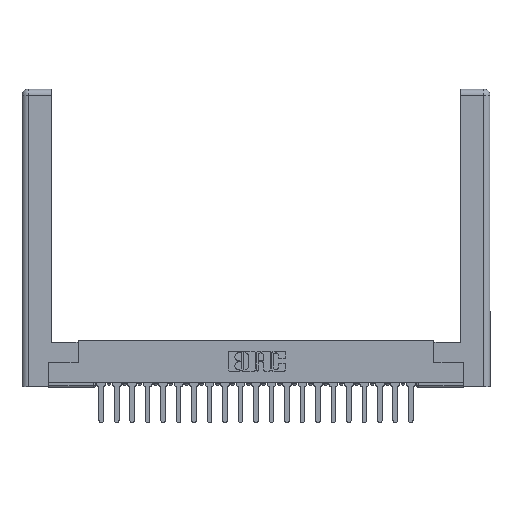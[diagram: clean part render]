
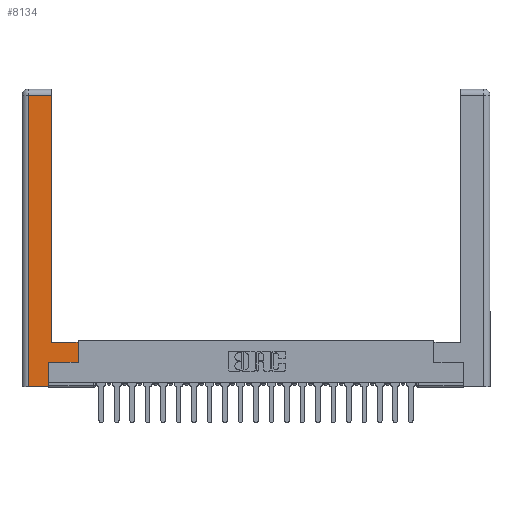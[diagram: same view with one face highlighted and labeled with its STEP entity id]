
A CAD part, top view. The second image highlights one B-rep face of the part: STEP entity #8134.
In plain terms, the highlighted planar face has unit normal (0, 0, 1).
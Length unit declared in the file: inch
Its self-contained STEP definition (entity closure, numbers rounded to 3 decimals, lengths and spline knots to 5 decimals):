
#376 = EDGE_CURVE ( 'NONE', #17551, #21999, #12902, .T. ) ;
#1391 = CARTESIAN_POINT ( 'NONE',  ( 0.295, 0.45, 0. ) ) ;
#1686 = LINE ( 'NONE', #14076, #10681 ) ;
#2041 = ORIENTED_EDGE ( 'NONE', *, *, #10246, .T. ) ;
#2140 = EDGE_LOOP ( 'NONE', ( #2041, #16626, #19138, #18649, #11762, #20562, #12938, #21196 ) ) ;
#3320 = VERTEX_POINT ( 'NONE', #7992 ) ;
#4151 = CARTESIAN_POINT ( 'NONE',  ( 0.565, 0.245, 0. ) ) ;
#4996 = VERTEX_POINT ( 'NONE', #14746 ) ;
#6112 = EDGE_CURVE ( 'NONE', #4996, #21614, #20547, .T. ) ;
#6127 = PLANE ( 'NONE',  #22877 ) ;
#6736 = VERTEX_POINT ( 'NONE', #1391 ) ;
#6826 = CARTESIAN_POINT ( 'NONE',  ( 0.265, 0.245, 0. ) ) ;
#7466 = VECTOR ( 'NONE', #13180, 39.37008 ) ;
#7992 = CARTESIAN_POINT ( 'NONE',  ( 0.565, 0.45, 0. ) ) ;
#8065 = EDGE_CURVE ( 'NONE', #11550, #17551, #21296, .T. ) ;
#8134 = ADVANCED_FACE ( 'NONE', ( #10956 ), #6127, .F. ) ;
#8315 = LINE ( 'NONE', #9216, #16371 ) ;
#8738 = LINE ( 'NONE', #15310, #21993 ) ;
#9216 = CARTESIAN_POINT ( 'NONE',  ( 0.265, 0., 0. ) ) ;
#9614 = CARTESIAN_POINT ( 'NONE',  ( 0.0615, 2.94, 0. ) ) ;
#9713 = DIRECTION ( 'NONE',  ( 0., 1., 0. ) ) ;
#9951 = DIRECTION ( 'NONE',  ( -1., 0., 0. ) ) ;
#10246 = EDGE_CURVE ( 'NONE', #6736, #23753, #1686, .T. ) ;
#10362 = LINE ( 'NONE', #9614, #7466 ) ;
#10661 = EDGE_CURVE ( 'NONE', #23753, #4996, #10362, .T. ) ;
#10681 = VECTOR ( 'NONE', #15895, 39.37008 ) ;
#10790 = VECTOR ( 'NONE', #16571, 39.37008 ) ;
#10956 = FACE_OUTER_BOUND ( 'NONE', #2140, .T. ) ;
#11110 = DIRECTION ( 'NONE',  ( -1., 0., 0. ) ) ;
#11181 = EDGE_CURVE ( 'NONE', #21614, #11550, #8315, .T. ) ;
#11276 = CARTESIAN_POINT ( 'NONE',  ( 0.295, 0.45, 0. ) ) ;
#11550 = VERTEX_POINT ( 'NONE', #19859 ) ;
#11762 = ORIENTED_EDGE ( 'NONE', *, *, #8065, .T. ) ;
#11785 = CARTESIAN_POINT ( 'NONE',  ( 0.265, 0.245, 0. ) ) ;
#12244 = CARTESIAN_POINT ( 'NONE',  ( 0.565, 0.245, 0. ) ) ;
#12902 = LINE ( 'NONE', #12244, #23511 ) ;
#12938 = ORIENTED_EDGE ( 'NONE', *, *, #23319, .T. ) ;
#13180 = DIRECTION ( 'NONE',  ( -1., 0., 0. ) ) ;
#14039 = CARTESIAN_POINT ( 'NONE',  ( 0.0615, 0., 0. ) ) ;
#14076 = CARTESIAN_POINT ( 'NONE',  ( 0.295, 3., 0. ) ) ;
#14661 = CARTESIAN_POINT ( 'NONE',  ( 0.0615, 0., 0. ) ) ;
#14746 = CARTESIAN_POINT ( 'NONE',  ( 0.0615, 2.94, 0. ) ) ;
#15310 = CARTESIAN_POINT ( 'NONE',  ( 0.565, 0.45, 0. ) ) ;
#15895 = DIRECTION ( 'NONE',  ( 0., 1., 0. ) ) ;
#16371 = VECTOR ( 'NONE', #22398, 39.37008 ) ;
#16571 = DIRECTION ( 'NONE',  ( 0., -1., 0. ) ) ;
#16626 = ORIENTED_EDGE ( 'NONE', *, *, #10661, .T. ) ;
#17202 = DIRECTION ( 'NONE',  ( 0., 1., 0. ) ) ;
#17239 = VECTOR ( 'NONE', #17202, 39.37008 ) ;
#17551 = VERTEX_POINT ( 'NONE', #6826 ) ;
#17882 = EDGE_CURVE ( 'NONE', #3320, #6736, #23026, .T. ) ;
#18074 = VECTOR ( 'NONE', #11110, 39.37008 ) ;
#18649 = ORIENTED_EDGE ( 'NONE', *, *, #11181, .T. ) ;
#18967 = DIRECTION ( 'NONE',  ( 0., 0., -1. ) ) ;
#19138 = ORIENTED_EDGE ( 'NONE', *, *, #6112, .T. ) ;
#19859 = CARTESIAN_POINT ( 'NONE',  ( 0.265, 0., 0. ) ) ;
#20547 = LINE ( 'NONE', #14661, #10790 ) ;
#20562 = ORIENTED_EDGE ( 'NONE', *, *, #376, .T. ) ;
#21196 = ORIENTED_EDGE ( 'NONE', *, *, #17882, .T. ) ;
#21296 = LINE ( 'NONE', #11785, #17239 ) ;
#21614 = VERTEX_POINT ( 'NONE', #14039 ) ;
#21715 = DIRECTION ( 'NONE',  ( 1., 0., 0. ) ) ;
#21993 = VECTOR ( 'NONE', #9713, 39.37008 ) ;
#21999 = VERTEX_POINT ( 'NONE', #4151 ) ;
#22398 = DIRECTION ( 'NONE',  ( 1., 0., 0. ) ) ;
#22877 = AXIS2_PLACEMENT_3D ( 'NONE', #22883, #18967, #9951 ) ;
#22883 = CARTESIAN_POINT ( 'NONE',  ( 0., 0., 0. ) ) ;
#23026 = LINE ( 'NONE', #11276, #18074 ) ;
#23319 = EDGE_CURVE ( 'NONE', #21999, #3320, #8738, .T. ) ;
#23511 = VECTOR ( 'NONE', #21715, 39.37008 ) ;
#23752 = CARTESIAN_POINT ( 'NONE',  ( 0.295, 2.94, 0. ) ) ;
#23753 = VERTEX_POINT ( 'NONE', #23752 ) ;
